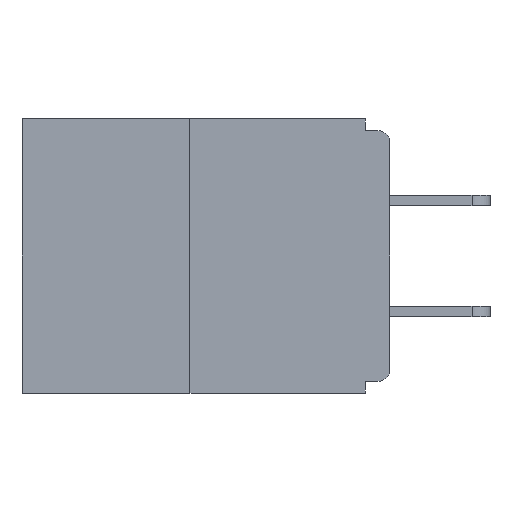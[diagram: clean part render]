
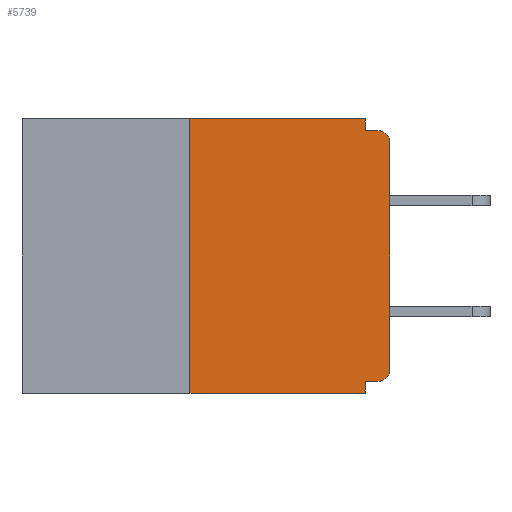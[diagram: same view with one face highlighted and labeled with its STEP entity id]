
A CAD part, left-side view. The second image highlights one B-rep face of the part: STEP entity #5739.
In plain terms, the highlighted planar face has unit normal (-1, 0, 0).
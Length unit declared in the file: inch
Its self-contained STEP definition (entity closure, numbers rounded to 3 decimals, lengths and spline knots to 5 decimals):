
#88 = DIRECTION ( 'NONE',  ( 0., 0., -1. ) ) ;
#1233 = VERTEX_POINT ( 'NONE', #4929 ) ;
#1653 = EDGE_CURVE ( 'NONE', #28365, #2746, #8394, .T. ) ;
#2746 = VERTEX_POINT ( 'NONE', #22973 ) ;
#2821 = CARTESIAN_POINT ( 'NONE',  ( 0., 0.015, -0.313 ) ) ;
#3065 = DIRECTION ( 'NONE',  ( 0., 0., -1. ) ) ;
#3727 = VECTOR ( 'NONE', #7872, 39.37008 ) ;
#4187 = DIRECTION ( 'NONE',  ( -1., 0., 0. ) ) ;
#4929 = CARTESIAN_POINT ( 'NONE',  ( 0., 0.031, -0.015 ) ) ;
#5255 = LINE ( 'NONE', #21820, #24222 ) ;
#5739 = ADVANCED_FACE ( 'NONE', ( #26592 ), #26277, .F. ) ;
#6417 = ORIENTED_EDGE ( 'NONE', *, *, #17431, .F. ) ;
#6500 = DIRECTION ( 'NONE',  ( 0., 0., 1. ) ) ;
#6559 = VECTOR ( 'NONE', #88, 39.37008 ) ;
#6567 = CARTESIAN_POINT ( 'NONE',  ( 0., 0.25, 0. ) ) ;
#6816 = CARTESIAN_POINT ( 'NONE',  ( 0., 0.015, -0.328 ) ) ;
#6940 = DIRECTION ( 'NONE',  ( 0., 0., -1. ) ) ;
#7443 = EDGE_CURVE ( 'NONE', #28365, #18257, #18134, .T. ) ;
#7627 = CARTESIAN_POINT ( 'NONE',  ( 0., 0.46, -0.343 ) ) ;
#7872 = DIRECTION ( 'NONE',  ( 0., 0., -1. ) ) ;
#7910 = CARTESIAN_POINT ( 'NONE',  ( 0., 0.25, -0.343 ) ) ;
#7950 = LINE ( 'NONE', #27364, #27624 ) ;
#8394 = LINE ( 'NONE', #7627, #26228 ) ;
#8518 = VECTOR ( 'NONE', #28325, 39.37008 ) ;
#8647 = EDGE_CURVE ( 'NONE', #18257, #17120, #5255, .T. ) ;
#9164 = EDGE_CURVE ( 'NONE', #27202, #21132, #26390, .T. ) ;
#9740 = VERTEX_POINT ( 'NONE', #26307 ) ;
#9749 = DIRECTION ( 'NONE',  ( -1., 0., 0. ) ) ;
#9818 = LINE ( 'NONE', #28304, #6559 ) ;
#9979 = LINE ( 'NONE', #12012, #8518 ) ;
#10451 = VECTOR ( 'NONE', #6500, 39.37008 ) ;
#10685 = AXIS2_PLACEMENT_3D ( 'NONE', #2821, #9749, #19168 ) ;
#11385 = LINE ( 'NONE', #28070, #3727 ) ;
#11928 = EDGE_LOOP ( 'NONE', ( #13699, #25705, #26630, #16429, #24067, #28714, #16230, #14089, #6417, #29613 ) ) ;
#11951 = CARTESIAN_POINT ( 'NONE',  ( 0., 0., -0.03 ) ) ;
#12012 = CARTESIAN_POINT ( 'NONE',  ( 0., 0., -0.328 ) ) ;
#12967 = DIRECTION ( 'NONE',  ( 0., 0., 1. ) ) ;
#13699 = ORIENTED_EDGE ( 'NONE', *, *, #8647, .F. ) ;
#14089 = ORIENTED_EDGE ( 'NONE', *, *, #9164, .T. ) ;
#14656 = EDGE_CURVE ( 'NONE', #17120, #1233, #9818, .T. ) ;
#14761 = VECTOR ( 'NONE', #12967, 39.37008 ) ;
#16230 = ORIENTED_EDGE ( 'NONE', *, *, #27518, .T. ) ;
#16429 = ORIENTED_EDGE ( 'NONE', *, *, #23429, .F. ) ;
#16769 = CARTESIAN_POINT ( 'NONE',  ( 0., 0.46, 0. ) ) ;
#17065 = DIRECTION ( 'NONE',  ( 1., 0., 0. ) ) ;
#17120 = VERTEX_POINT ( 'NONE', #25768 ) ;
#17431 = EDGE_CURVE ( 'NONE', #1233, #21132, #7950, .T. ) ;
#18085 = VERTEX_POINT ( 'NONE', #21531 ) ;
#18134 = LINE ( 'NONE', #25434, #10451 ) ;
#18257 = VERTEX_POINT ( 'NONE', #6567 ) ;
#19168 = DIRECTION ( 'NONE',  ( 0., 0., -1. ) ) ;
#19416 = AXIS2_PLACEMENT_3D ( 'NONE', #20944, #4187, #6940 ) ;
#19643 = CARTESIAN_POINT ( 'NONE',  ( 0., 0., 0. ) ) ;
#20619 = DIRECTION ( 'NONE',  ( 0., -1., 0. ) ) ;
#20944 = CARTESIAN_POINT ( 'NONE',  ( 0., 0.015, -0.03 ) ) ;
#21132 = VERTEX_POINT ( 'NONE', #29048 ) ;
#21531 = CARTESIAN_POINT ( 'NONE',  ( 0., 0.031, -0.328 ) ) ;
#21820 = CARTESIAN_POINT ( 'NONE',  ( 0., 0.46, 0. ) ) ;
#22973 = CARTESIAN_POINT ( 'NONE',  ( 0., 0.031, -0.343 ) ) ;
#23408 = AXIS2_PLACEMENT_3D ( 'NONE', #16769, #17065, #3065 ) ;
#23429 = EDGE_CURVE ( 'NONE', #18085, #2746, #11385, .T. ) ;
#24067 = ORIENTED_EDGE ( 'NONE', *, *, #29465, .F. ) ;
#24104 = EDGE_CURVE ( 'NONE', #25091, #9740, #25167, .T. ) ;
#24222 = VECTOR ( 'NONE', #26136, 39.37008 ) ;
#24943 = LINE ( 'NONE', #19643, #14761 ) ;
#25091 = VERTEX_POINT ( 'NONE', #6816 ) ;
#25167 = CIRCLE ( 'NONE', #10685, 0.015 ) ;
#25434 = CARTESIAN_POINT ( 'NONE',  ( 0., 0.25, 0. ) ) ;
#25705 = ORIENTED_EDGE ( 'NONE', *, *, #7443, .F. ) ;
#25768 = CARTESIAN_POINT ( 'NONE',  ( 0., 0.031, 0. ) ) ;
#26136 = DIRECTION ( 'NONE',  ( 0., -1., 0. ) ) ;
#26228 = VECTOR ( 'NONE', #28326, 39.37008 ) ;
#26277 = PLANE ( 'NONE',  #23408 ) ;
#26307 = CARTESIAN_POINT ( 'NONE',  ( 0., 0., -0.313 ) ) ;
#26390 = CIRCLE ( 'NONE', #19416, 0.015 ) ;
#26592 = FACE_OUTER_BOUND ( 'NONE', #11928, .T. ) ;
#26630 = ORIENTED_EDGE ( 'NONE', *, *, #1653, .T. ) ;
#27202 = VERTEX_POINT ( 'NONE', #11951 ) ;
#27364 = CARTESIAN_POINT ( 'NONE',  ( 0., 0., -0.015 ) ) ;
#27518 = EDGE_CURVE ( 'NONE', #9740, #27202, #24943, .T. ) ;
#27624 = VECTOR ( 'NONE', #20619, 39.37008 ) ;
#28070 = CARTESIAN_POINT ( 'NONE',  ( 0., 0.031, -0.343 ) ) ;
#28304 = CARTESIAN_POINT ( 'NONE',  ( 0., 0.031, 0. ) ) ;
#28325 = DIRECTION ( 'NONE',  ( 0., 1., 0. ) ) ;
#28326 = DIRECTION ( 'NONE',  ( 0., -1., 0. ) ) ;
#28365 = VERTEX_POINT ( 'NONE', #7910 ) ;
#28714 = ORIENTED_EDGE ( 'NONE', *, *, #24104, .T. ) ;
#29048 = CARTESIAN_POINT ( 'NONE',  ( 0., 0.015, -0.015 ) ) ;
#29465 = EDGE_CURVE ( 'NONE', #25091, #18085, #9979, .T. ) ;
#29613 = ORIENTED_EDGE ( 'NONE', *, *, #14656, .F. ) ;
